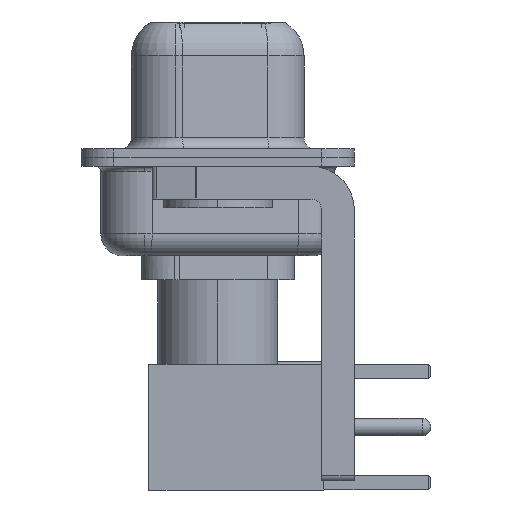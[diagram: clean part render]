
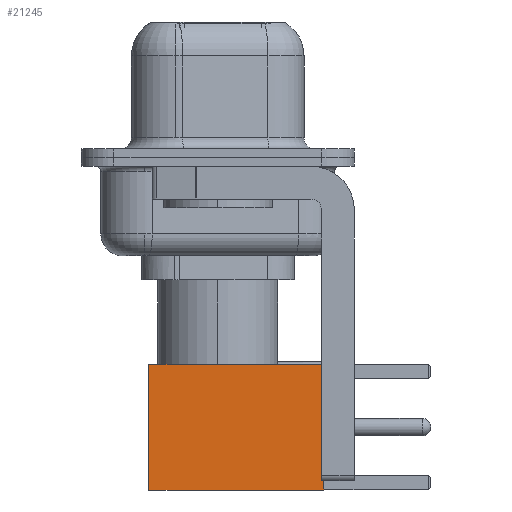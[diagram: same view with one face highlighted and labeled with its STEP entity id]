
A CAD part, left-side view. The second image highlights one B-rep face of the part: STEP entity #21245.
In plain terms, the highlighted face is planar.
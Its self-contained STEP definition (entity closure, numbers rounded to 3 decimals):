
#108 = ORIENTED_EDGE ( 'NONE', *, *, #3617, .F. ) ;
#133 = ORIENTED_EDGE ( 'NONE', *, *, #5233, .T. ) ;
#250 = DIRECTION ( 'NONE',  ( 0., 0., -1. ) ) ;
#921 = EDGE_CURVE ( 'NONE', #24416, #10082, #13806, .T. ) ;
#3617 = EDGE_CURVE ( 'NONE', #24416, #9102, #18102, .T. ) ;
#3657 = DIRECTION ( 'NONE',  ( 0., 0., -1. ) ) ;
#4913 = CARTESIAN_POINT ( 'NONE',  ( 0., 2.875, 8. ) ) ;
#5201 = DIRECTION ( 'NONE',  ( 0., 0., 1. ) ) ;
#5233 = EDGE_CURVE ( 'NONE', #10082, #18781, #17219, .T. ) ;
#5264 = CARTESIAN_POINT ( 'NONE',  ( -2.875, 2.875, 0. ) ) ;
#7537 = ORIENTED_EDGE ( 'NONE', *, *, #921, .T. ) ;
#8710 = VECTOR ( 'NONE', #11923, 1000. ) ;
#9102 = VERTEX_POINT ( 'NONE', #26586 ) ;
#9352 = EDGE_CURVE ( 'NONE', #9102, #18781, #11845, .T. ) ;
#10082 = VERTEX_POINT ( 'NONE', #17497 ) ;
#11668 = FACE_OUTER_BOUND ( 'NONE', #19372, .T. ) ;
#11845 = LINE ( 'NONE', #14540, #24070 ) ;
#11923 = DIRECTION ( 'NONE',  ( -1., 0., 0. ) ) ;
#13806 = LINE ( 'NONE', #17563, #25275 ) ;
#13875 = CARTESIAN_POINT ( 'NONE',  ( 2.875, 2.875, 8. ) ) ;
#14540 = CARTESIAN_POINT ( 'NONE',  ( -2.875, 2.875, 0. ) ) ;
#15799 = VECTOR ( 'NONE', #24230, 1000. ) ;
#16089 = PLANE ( 'NONE',  #20167 ) ;
#17219 = LINE ( 'NONE', #23798, #15799 ) ;
#17497 = CARTESIAN_POINT ( 'NONE',  ( 2.875, 2.875, 0. ) ) ;
#17563 = CARTESIAN_POINT ( 'NONE',  ( 2.875, 2.875, 0. ) ) ;
#17676 = ORIENTED_EDGE ( 'NONE', *, *, #9352, .F. ) ;
#18102 = LINE ( 'NONE', #4913, #8710 ) ;
#18781 = VERTEX_POINT ( 'NONE', #5264 ) ;
#19372 = EDGE_LOOP ( 'NONE', ( #7537, #133, #17676, #108 ) ) ;
#20167 = AXIS2_PLACEMENT_3D ( 'NONE', #20379, #24825, #5201 ) ;
#20379 = CARTESIAN_POINT ( 'NONE',  ( 2.875, 2.875, 0. ) ) ;
#21245 = ADVANCED_FACE ( 'NONE', ( #11668 ), #16089, .T. ) ;
#23798 = CARTESIAN_POINT ( 'NONE',  ( 0., 2.875, 0. ) ) ;
#24070 = VECTOR ( 'NONE', #3657, 1000. ) ;
#24230 = DIRECTION ( 'NONE',  ( -1., 0., 0. ) ) ;
#24416 = VERTEX_POINT ( 'NONE', #13875 ) ;
#24825 = DIRECTION ( 'NONE',  ( 0., 1., 0. ) ) ;
#25275 = VECTOR ( 'NONE', #250, 1000. ) ;
#26586 = CARTESIAN_POINT ( 'NONE',  ( -2.875, 2.875, 8. ) ) ;
